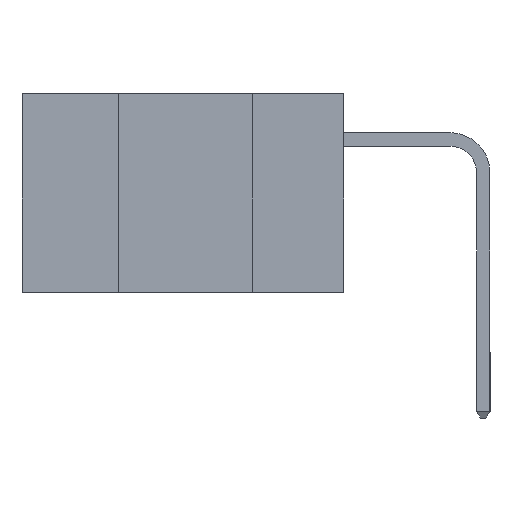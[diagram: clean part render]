
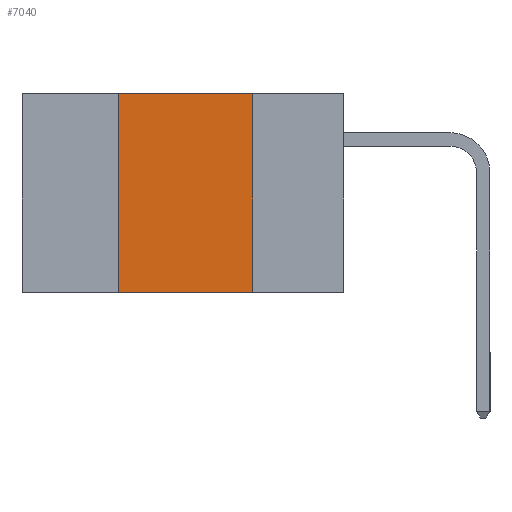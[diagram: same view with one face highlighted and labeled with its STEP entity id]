
A CAD part, left-side view. The second image highlights one B-rep face of the part: STEP entity #7040.
In plain terms, the highlighted planar face has unit normal (-1, 0, 0).
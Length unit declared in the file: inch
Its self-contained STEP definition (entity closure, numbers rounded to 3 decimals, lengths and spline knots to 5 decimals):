
#183 = CARTESIAN_POINT ( 'NONE',  ( 0., 0.17, 0. ) ) ;
#241 = ORIENTED_EDGE ( 'NONE', *, *, #5302, .T. ) ;
#775 = EDGE_CURVE ( 'NONE', #8572, #8980, #9350, .T. ) ;
#778 = DIRECTION ( 'NONE',  ( 0., 0., -1. ) ) ;
#822 = AXIS2_PLACEMENT_3D ( 'NONE', #7174, #6291, #2569 ) ;
#1468 = LINE ( 'NONE', #3776, #6645 ) ;
#1630 = ORIENTED_EDGE ( 'NONE', *, *, #2470, .F. ) ;
#2000 = FACE_OUTER_BOUND ( 'NONE', #5740, .T. ) ;
#2279 = CARTESIAN_POINT ( 'NONE',  ( 0., 0.17, 0. ) ) ;
#2308 = DIRECTION ( 'NONE',  ( 0., -1., 0. ) ) ;
#2470 = EDGE_CURVE ( 'NONE', #6963, #9355, #9656, .T. ) ;
#2569 = DIRECTION ( 'NONE',  ( 0., 0., -1. ) ) ;
#2985 = CARTESIAN_POINT ( 'NONE',  ( 0., 0.42, -0.37 ) ) ;
#3272 = VECTOR ( 'NONE', #7783, 39.37008 ) ;
#3338 = VECTOR ( 'NONE', #5122, 39.37008 ) ;
#3592 = ORIENTED_EDGE ( 'NONE', *, *, #8369, .F. ) ;
#3776 = CARTESIAN_POINT ( 'NONE',  ( 0., 0.6, -0.37 ) ) ;
#4984 = VECTOR ( 'NONE', #778, 39.37008 ) ;
#5122 = DIRECTION ( 'NONE',  ( 0., 0., 1. ) ) ;
#5302 = EDGE_CURVE ( 'NONE', #8572, #9355, #1468, .T. ) ;
#5608 = CARTESIAN_POINT ( 'NONE',  ( 0., 0.6, 0. ) ) ;
#5740 = EDGE_LOOP ( 'NONE', ( #1630, #3592, #6320, #241 ) ) ;
#6291 = DIRECTION ( 'NONE',  ( 1., 0., 0. ) ) ;
#6320 = ORIENTED_EDGE ( 'NONE', *, *, #775, .F. ) ;
#6507 = CARTESIAN_POINT ( 'NONE',  ( 0., 0.17, -0.37 ) ) ;
#6645 = VECTOR ( 'NONE', #2308, 39.37008 ) ;
#6963 = VERTEX_POINT ( 'NONE', #183 ) ;
#7040 = ADVANCED_FACE ( 'NONE', ( #2000 ), #7947, .F. ) ;
#7174 = CARTESIAN_POINT ( 'NONE',  ( 0., 0.6, 0. ) ) ;
#7492 = CARTESIAN_POINT ( 'NONE',  ( 0., 0.42, 0. ) ) ;
#7730 = CARTESIAN_POINT ( 'NONE',  ( 0., 0.42, 0. ) ) ;
#7783 = DIRECTION ( 'NONE',  ( 0., -1., 0. ) ) ;
#7947 = PLANE ( 'NONE',  #822 ) ;
#8306 = LINE ( 'NONE', #5608, #3272 ) ;
#8369 = EDGE_CURVE ( 'NONE', #8980, #6963, #8306, .T. ) ;
#8572 = VERTEX_POINT ( 'NONE', #2985 ) ;
#8980 = VERTEX_POINT ( 'NONE', #7730 ) ;
#9350 = LINE ( 'NONE', #7492, #3338 ) ;
#9355 = VERTEX_POINT ( 'NONE', #6507 ) ;
#9656 = LINE ( 'NONE', #2279, #4984 ) ;
